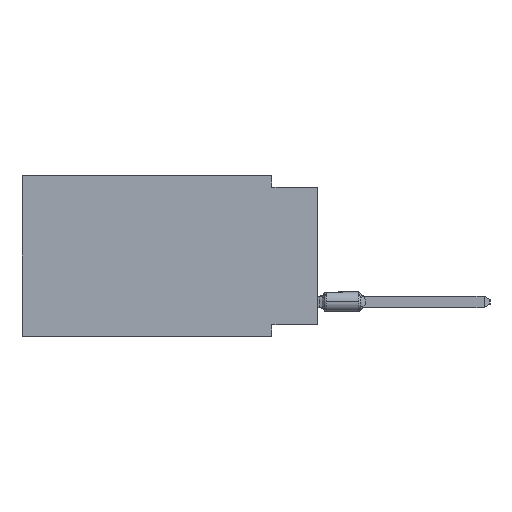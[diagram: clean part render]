
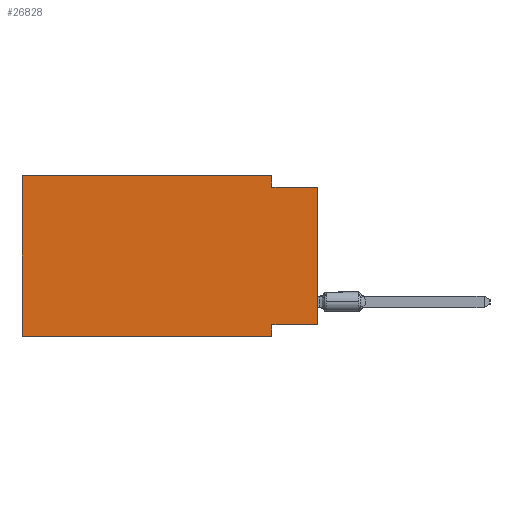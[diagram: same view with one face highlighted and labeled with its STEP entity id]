
A CAD part, left-side view. The second image highlights one B-rep face of the part: STEP entity #26828.
In plain terms, the highlighted planar face has unit normal (-1, 0, 0).
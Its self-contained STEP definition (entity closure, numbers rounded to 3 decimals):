
#632 = LINE ( 'NONE', #2950, #21848 ) ;
#1393 = CARTESIAN_POINT ( 'NONE',  ( 0., 2.54, -0.635 ) ) ;
#1531 = CARTESIAN_POINT ( 'NONE',  ( 0., 2.54, -8.89 ) ) ;
#2491 = EDGE_CURVE ( 'NONE', #24244, #34719, #4238, .T. ) ;
#2950 = CARTESIAN_POINT ( 'NONE',  ( 0., 0., -8.255 ) ) ;
#2995 = CARTESIAN_POINT ( 'NONE',  ( 0., 0., 0. ) ) ;
#3348 = CARTESIAN_POINT ( 'NONE',  ( 0., 16.383, 0. ) ) ;
#3535 = LINE ( 'NONE', #3348, #16648 ) ;
#3744 = CARTESIAN_POINT ( 'NONE',  ( 0., 16.383, 0. ) ) ;
#4175 = ORIENTED_EDGE ( 'NONE', *, *, #9810, .T. ) ;
#4238 = LINE ( 'NONE', #1531, #30370 ) ;
#4453 = EDGE_CURVE ( 'NONE', #6750, #22691, #20794, .T. ) ;
#4620 = CARTESIAN_POINT ( 'NONE',  ( 0., 0., -8.255 ) ) ;
#5088 = LINE ( 'NONE', #26330, #30673 ) ;
#5445 = VECTOR ( 'NONE', #6442, 1000. ) ;
#6390 = LINE ( 'NONE', #14914, #31285 ) ;
#6442 = DIRECTION ( 'NONE',  ( 0., 0., 1. ) ) ;
#6578 = DIRECTION ( 'NONE',  ( 0., -1., 0. ) ) ;
#6750 = VERTEX_POINT ( 'NONE', #1393 ) ;
#6778 = CARTESIAN_POINT ( 'NONE',  ( 0., 16.383, 0. ) ) ;
#9142 = VERTEX_POINT ( 'NONE', #13294 ) ;
#9810 = EDGE_CURVE ( 'NONE', #31899, #22691, #24235, .T. ) ;
#13294 = CARTESIAN_POINT ( 'NONE',  ( 0., 2.54, 0. ) ) ;
#13614 = VECTOR ( 'NONE', #26229, 1000. ) ;
#13810 = EDGE_CURVE ( 'NONE', #31899, #24244, #632, .T. ) ;
#14585 = ORIENTED_EDGE ( 'NONE', *, *, #13810, .F. ) ;
#14728 = DIRECTION ( 'NONE',  ( 0., -1., 0. ) ) ;
#14914 = CARTESIAN_POINT ( 'NONE',  ( 0., 16.383, 0. ) ) ;
#15108 = EDGE_LOOP ( 'NONE', ( #4175, #20265, #34958, #26467, #22940, #24383, #17971, #14585 ) ) ;
#16648 = VECTOR ( 'NONE', #27313, 1000. ) ;
#17706 = CARTESIAN_POINT ( 'NONE',  ( 0., 0., -0.635 ) ) ;
#17920 = CARTESIAN_POINT ( 'NONE',  ( 0., 2.54, -8.255 ) ) ;
#17971 = ORIENTED_EDGE ( 'NONE', *, *, #2491, .F. ) ;
#18703 = LINE ( 'NONE', #25289, #19681 ) ;
#19091 = DIRECTION ( 'NONE',  ( 0., 0., -1. ) ) ;
#19681 = VECTOR ( 'NONE', #19091, 1000. ) ;
#20265 = ORIENTED_EDGE ( 'NONE', *, *, #4453, .F. ) ;
#20794 = LINE ( 'NONE', #17706, #13614 ) ;
#21848 = VECTOR ( 'NONE', #23808, 1000. ) ;
#22602 = AXIS2_PLACEMENT_3D ( 'NONE', #6778, #23612, #32683 ) ;
#22691 = VERTEX_POINT ( 'NONE', #36854 ) ;
#22940 = ORIENTED_EDGE ( 'NONE', *, *, #30338, .F. ) ;
#23212 = EDGE_CURVE ( 'NONE', #25732, #34719, #5088, .T. ) ;
#23301 = CARTESIAN_POINT ( 'NONE',  ( 0., 16.383, -8.89 ) ) ;
#23612 = DIRECTION ( 'NONE',  ( 1., 0., 0. ) ) ;
#23808 = DIRECTION ( 'NONE',  ( 0., 1., 0. ) ) ;
#24235 = LINE ( 'NONE', #2995, #5445 ) ;
#24244 = VERTEX_POINT ( 'NONE', #17920 ) ;
#24383 = ORIENTED_EDGE ( 'NONE', *, *, #23212, .T. ) ;
#25289 = CARTESIAN_POINT ( 'NONE',  ( 0., 2.54, 0. ) ) ;
#25732 = VERTEX_POINT ( 'NONE', #23301 ) ;
#26229 = DIRECTION ( 'NONE',  ( 0., -1., 0. ) ) ;
#26330 = CARTESIAN_POINT ( 'NONE',  ( 0., 16.383, -8.89 ) ) ;
#26467 = ORIENTED_EDGE ( 'NONE', *, *, #28021, .F. ) ;
#26828 = ADVANCED_FACE ( 'NONE', ( #32858 ), #32479, .F. ) ;
#27313 = DIRECTION ( 'NONE',  ( 0., 0., 1. ) ) ;
#28021 = EDGE_CURVE ( 'NONE', #36581, #9142, #6390, .T. ) ;
#30338 = EDGE_CURVE ( 'NONE', #25732, #36581, #3535, .T. ) ;
#30370 = VECTOR ( 'NONE', #30700, 1000. ) ;
#30673 = VECTOR ( 'NONE', #14728, 1000. ) ;
#30700 = DIRECTION ( 'NONE',  ( 0., 0., -1. ) ) ;
#31285 = VECTOR ( 'NONE', #6578, 1000. ) ;
#31899 = VERTEX_POINT ( 'NONE', #4620 ) ;
#32389 = CARTESIAN_POINT ( 'NONE',  ( 0., 2.54, -8.89 ) ) ;
#32479 = PLANE ( 'NONE',  #22602 ) ;
#32683 = DIRECTION ( 'NONE',  ( 0., 0., -1. ) ) ;
#32858 = FACE_OUTER_BOUND ( 'NONE', #15108, .T. ) ;
#34719 = VERTEX_POINT ( 'NONE', #32389 ) ;
#34958 = ORIENTED_EDGE ( 'NONE', *, *, #35744, .F. ) ;
#35744 = EDGE_CURVE ( 'NONE', #9142, #6750, #18703, .T. ) ;
#36581 = VERTEX_POINT ( 'NONE', #3744 ) ;
#36854 = CARTESIAN_POINT ( 'NONE',  ( 0., 0., -0.635 ) ) ;
